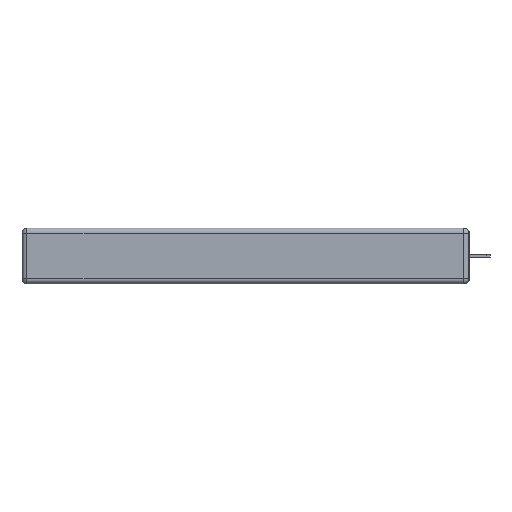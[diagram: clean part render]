
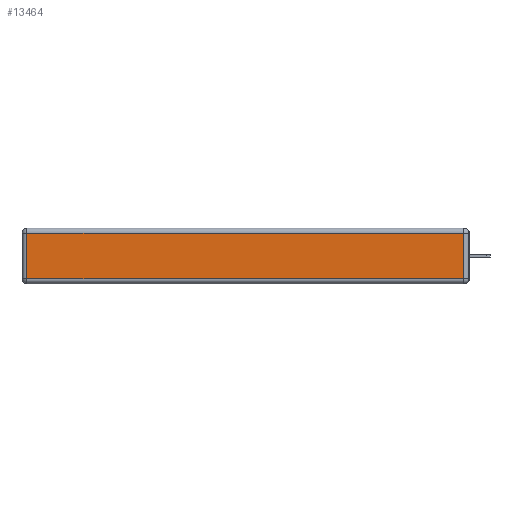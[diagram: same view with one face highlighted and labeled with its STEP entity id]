
A CAD part, left-side view. The second image highlights one B-rep face of the part: STEP entity #13464.
In plain terms, the highlighted planar face has unit normal (-1, 0, 0).
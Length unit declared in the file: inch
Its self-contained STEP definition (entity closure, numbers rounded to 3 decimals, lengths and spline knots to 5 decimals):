
#1029 = CARTESIAN_POINT ( 'NONE',  ( 0., 0., -0.343 ) ) ;
#1059 = ORIENTED_EDGE ( 'NONE', *, *, #3100, .T. ) ;
#2541 = ORIENTED_EDGE ( 'NONE', *, *, #6006, .T. ) ;
#3100 = EDGE_CURVE ( 'NONE', #10833, #15332, #4118, .T. ) ;
#3447 = DIRECTION ( 'NONE',  ( 0., 0., 1. ) ) ;
#3649 = DIRECTION ( 'NONE',  ( 0., 0., 1. ) ) ;
#4111 = VECTOR ( 'NONE', #14342, 39.37008 ) ;
#4118 = LINE ( 'NONE', #14112, #16042 ) ;
#5694 = ORIENTED_EDGE ( 'NONE', *, *, #6565, .T. ) ;
#6006 = EDGE_CURVE ( 'NONE', #15332, #6872, #6557, .T. ) ;
#6457 = FACE_OUTER_BOUND ( 'NONE', #11322, .T. ) ;
#6557 = LINE ( 'NONE', #9334, #4111 ) ;
#6565 = EDGE_CURVE ( 'NONE', #6872, #13394, #8332, .T. ) ;
#6872 = VERTEX_POINT ( 'NONE', #11617 ) ;
#7106 = CARTESIAN_POINT ( 'NONE',  ( 0., 0.03, -0.343 ) ) ;
#7271 = CARTESIAN_POINT ( 'NONE',  ( 0., 2.72, -0.03 ) ) ;
#8332 = LINE ( 'NONE', #14409, #13796 ) ;
#9334 = CARTESIAN_POINT ( 'NONE',  ( 0., 2.72, -0.343 ) ) ;
#9483 = DIRECTION ( 'NONE',  ( 0., -1., 0. ) ) ;
#10705 = LINE ( 'NONE', #7106, #14404 ) ;
#10833 = VERTEX_POINT ( 'NONE', #13262 ) ;
#11218 = EDGE_CURVE ( 'NONE', #13394, #10833, #10705, .T. ) ;
#11322 = EDGE_LOOP ( 'NONE', ( #5694, #13740, #1059, #2541 ) ) ;
#11617 = CARTESIAN_POINT ( 'NONE',  ( 0., 2.72, -0.313 ) ) ;
#12883 = DIRECTION ( 'NONE',  ( 0., 1., 0. ) ) ;
#13262 = CARTESIAN_POINT ( 'NONE',  ( 0., 0.03, -0.03 ) ) ;
#13394 = VERTEX_POINT ( 'NONE', #15609 ) ;
#13464 = ADVANCED_FACE ( 'NONE', ( #6457 ), #15174, .T. ) ;
#13648 = AXIS2_PLACEMENT_3D ( 'NONE', #1029, #15940, #3649 ) ;
#13740 = ORIENTED_EDGE ( 'NONE', *, *, #11218, .T. ) ;
#13796 = VECTOR ( 'NONE', #9483, 39.37008 ) ;
#14112 = CARTESIAN_POINT ( 'NONE',  ( 0., 2.75, -0.03 ) ) ;
#14342 = DIRECTION ( 'NONE',  ( 0., 0., -1. ) ) ;
#14404 = VECTOR ( 'NONE', #3447, 39.37008 ) ;
#14409 = CARTESIAN_POINT ( 'NONE',  ( 0., 0., -0.313 ) ) ;
#15174 = PLANE ( 'NONE',  #13648 ) ;
#15332 = VERTEX_POINT ( 'NONE', #7271 ) ;
#15609 = CARTESIAN_POINT ( 'NONE',  ( 0., 0.03, -0.313 ) ) ;
#15940 = DIRECTION ( 'NONE',  ( -1., 0., 0. ) ) ;
#16042 = VECTOR ( 'NONE', #12883, 39.37008 ) ;
